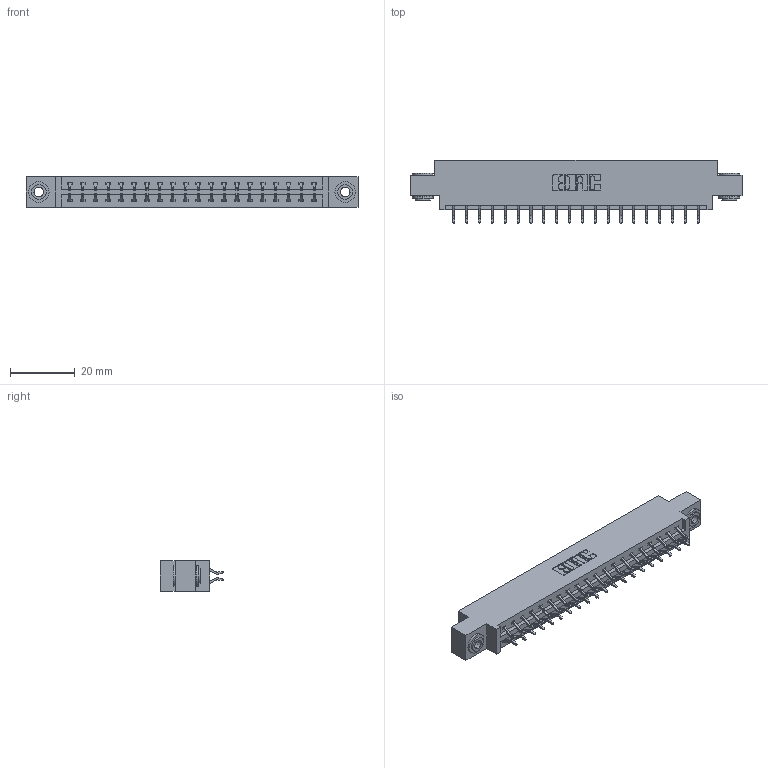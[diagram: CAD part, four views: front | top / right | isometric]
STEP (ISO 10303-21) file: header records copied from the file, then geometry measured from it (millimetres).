
FILE_DESCRIPTION (( 'STEP AP203' ), '1' );
FILE_NAME ('337-040-556-803.STEP', '2018-08-08T20:22:49', ( '' ), ( '' ), 'SwSTEP 2.0', 'SolidWorks 2016', '' );
FILE_SCHEMA (( 'CONFIG_CONTROL_DESIGN' ));
Length unit declared in the file: inch
Products named in the file (4): 345-250-002_345-250-002-102; 337-040-556-803; 337 Part_0.170 Offset - 0.156 Dia-TH; 345-292-001_556 Tail
Assembly tree (43 placements, depth 2):
  337-040-556-803
    337 Part_0.170 Offset - 0.156 Dia-TH
    345-292-001_556 Tail  x40
    345-250-002_345-250-002-102  x2
Bounding box: 102.26 x 19.57 x 9.4 mm (x, y, z)
Volume: 10384.5 mm3; surface area: 11816 mm2
Topology: 43 solids, 43 shells, 2556 faces, 7559 edges, 4982 vertices
Faces by surface type: plane 1764, cylinder 784, cone 8
Entity records: 19354 total; most frequent: CARTESIAN_POINT 3269, ORIENTED_EDGE 3186, DIRECTION 2843, EDGE_CURVE 1593, VECTOR 1433, LINE 1433, VERTEX_POINT 1058, AXIS2_PLACEMENT_3D 705
